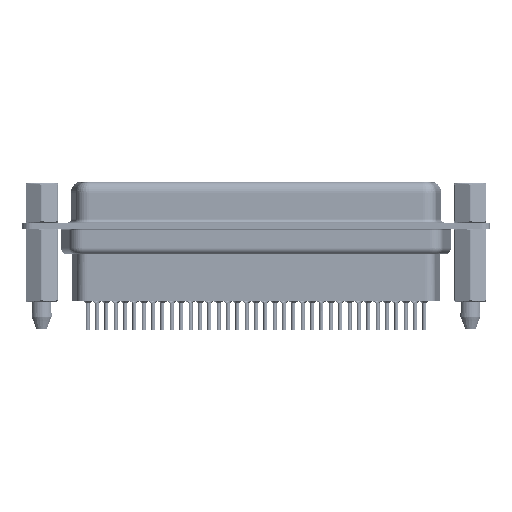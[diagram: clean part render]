
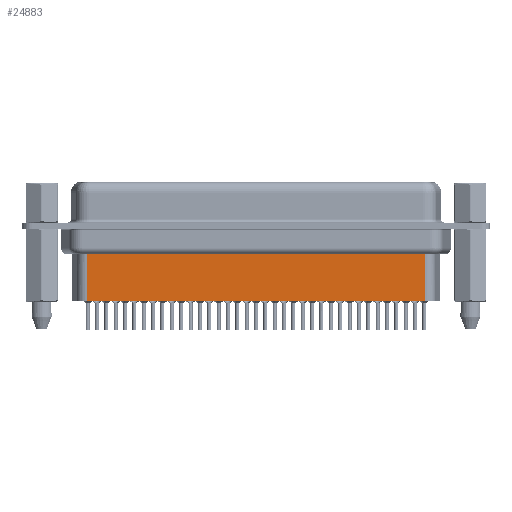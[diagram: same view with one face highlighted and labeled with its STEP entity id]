
A CAD part, front view. The second image highlights one B-rep face of the part: STEP entity #24883.
In plain terms, the highlighted planar face has unit normal (0, -1, 0).
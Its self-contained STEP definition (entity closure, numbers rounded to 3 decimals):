
#571 = CARTESIAN_POINT ( 'NONE',  ( 6.706, -3.5, -11.15 ) ) ;
#640 = ORIENTED_EDGE ( 'NONE', *, *, #25460, .T. ) ;
#1453 = VECTOR ( 'NONE', #3455, 1000. ) ;
#3455 = DIRECTION ( 'NONE',  ( 0., 0., -1. ) ) ;
#3700 = LINE ( 'NONE', #29312, #35901 ) ;
#6994 = CARTESIAN_POINT ( 'NONE',  ( 56.794, -3.5, -11.15 ) ) ;
#7204 = LINE ( 'NONE', #7811, #36616 ) ;
#7811 = CARTESIAN_POINT ( 'NONE',  ( 6.459, -3.5, -4.097 ) ) ;
#9708 = EDGE_CURVE ( 'NONE', #21311, #30045, #27121, .T. ) ;
#10541 = DIRECTION ( 'NONE',  ( -1., 0., 0. ) ) ;
#11228 = CARTESIAN_POINT ( 'NONE',  ( 6.706, -3.5, -3.1 ) ) ;
#14388 = FACE_OUTER_BOUND ( 'NONE', #18579, .T. ) ;
#14683 = ORIENTED_EDGE ( 'NONE', *, *, #9708, .F. ) ;
#15272 = VERTEX_POINT ( 'NONE', #18625 ) ;
#16173 = CARTESIAN_POINT ( 'NONE',  ( 6.706, -3.5, -11.15 ) ) ;
#17103 = VECTOR ( 'NONE', #26418, 1000. ) ;
#18579 = EDGE_LOOP ( 'NONE', ( #14683, #34107, #640, #37279 ) ) ;
#18625 = CARTESIAN_POINT ( 'NONE',  ( 6.706, -3.5, -4.097 ) ) ;
#19314 = CARTESIAN_POINT ( 'NONE',  ( 56.794, -3.5, -3.1 ) ) ;
#20819 = DIRECTION ( 'NONE',  ( 1., 0., 0. ) ) ;
#21311 = VERTEX_POINT ( 'NONE', #39807 ) ;
#24883 = ADVANCED_FACE ( 'NONE', ( #14388 ), #29967, .T. ) ;
#25460 = EDGE_CURVE ( 'NONE', #15272, #34216, #3700, .T. ) ;
#26030 = EDGE_CURVE ( 'NONE', #21311, #15272, #7204, .T. ) ;
#26418 = DIRECTION ( 'NONE',  ( -1., 0., 0. ) ) ;
#26449 = DIRECTION ( 'NONE',  ( 0., -1., 0. ) ) ;
#27121 = LINE ( 'NONE', #19314, #1453 ) ;
#29111 = DIRECTION ( 'NONE',  ( 0., 0., -1. ) ) ;
#29312 = CARTESIAN_POINT ( 'NONE',  ( 6.706, -3.5, -3.1 ) ) ;
#29967 = PLANE ( 'NONE',  #33853 ) ;
#30045 = VERTEX_POINT ( 'NONE', #6994 ) ;
#33251 = LINE ( 'NONE', #571, #17103 ) ;
#33853 = AXIS2_PLACEMENT_3D ( 'NONE', #11228, #26449, #20819 ) ;
#34107 = ORIENTED_EDGE ( 'NONE', *, *, #26030, .T. ) ;
#34216 = VERTEX_POINT ( 'NONE', #16173 ) ;
#35901 = VECTOR ( 'NONE', #29111, 1000. ) ;
#36399 = EDGE_CURVE ( 'NONE', #30045, #34216, #33251, .T. ) ;
#36616 = VECTOR ( 'NONE', #10541, 1000. ) ;
#37279 = ORIENTED_EDGE ( 'NONE', *, *, #36399, .F. ) ;
#39807 = CARTESIAN_POINT ( 'NONE',  ( 56.794, -3.5, -4.097 ) ) ;
